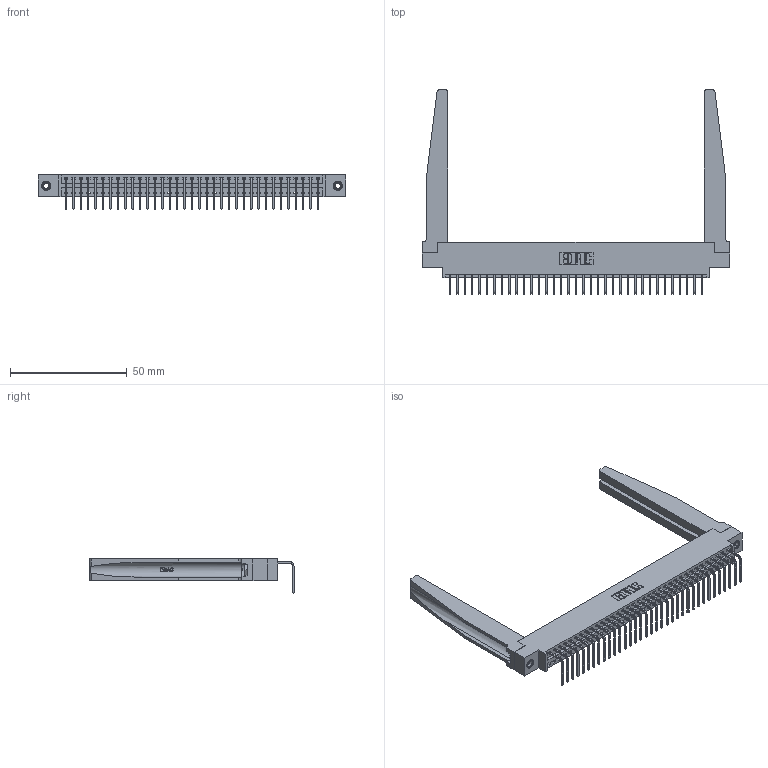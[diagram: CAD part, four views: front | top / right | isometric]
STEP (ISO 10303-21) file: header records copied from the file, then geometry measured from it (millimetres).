
FILE_DESCRIPTION (( 'STEP AP203' ), '1' );
FILE_NAME ('346-035-558-678.STEP', '2022-05-06T23:48:13', ( '' ), ( '' ), 'SwSTEP 2.0', 'SolidWorks 2020', '' );
FILE_SCHEMA (( 'CONFIG_CONTROL_DESIGN' ));
Length unit declared in the file: inch
Products named in the file (5): 345-292-001_558 Tail - 2; 346-035-558-678; 346 Part_0.170 Offset - 0.156 Dia-TH; 346-220-078_345-220-078; 345-250-001_345-250-001-102
Assembly tree (40 placements, depth 2):
  346-035-558-678
    346 Part_0.170 Offset - 0.156 Dia-TH
    345-292-001_558 Tail - 2  x35
    346-220-078_345-220-078  x2
    345-250-001_345-250-001-102  x2
Bounding box: 131.7 x 87.44 x 14.73 mm (x, y, z)
Volume: 19411 mm3; surface area: 22979 mm2
Topology: 40 solids, 40 shells, 2474 faces, 7355 edges, 4846 vertices
Faces by surface type: plane 1706, cylinder 716, bspline 36, cone 12, torus 4
Entity records: 28044 total; most frequent: CARTESIAN_POINT 5726, ORIENTED_EDGE 4582, DIRECTION 4043, EDGE_CURVE 2291, VECTOR 1925, LINE 1925, VERTEX_POINT 1520, AXIS2_PLACEMENT_3D 1059
